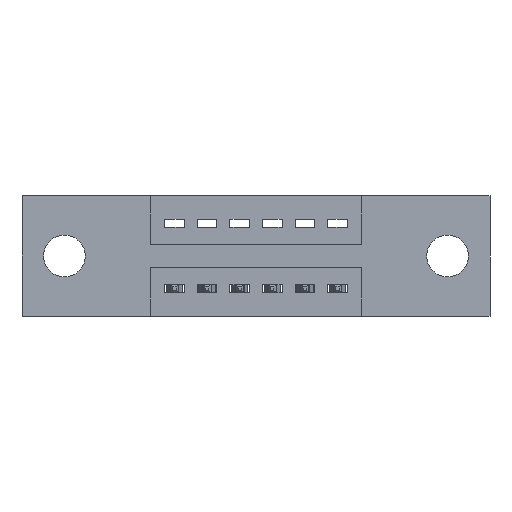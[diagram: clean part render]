
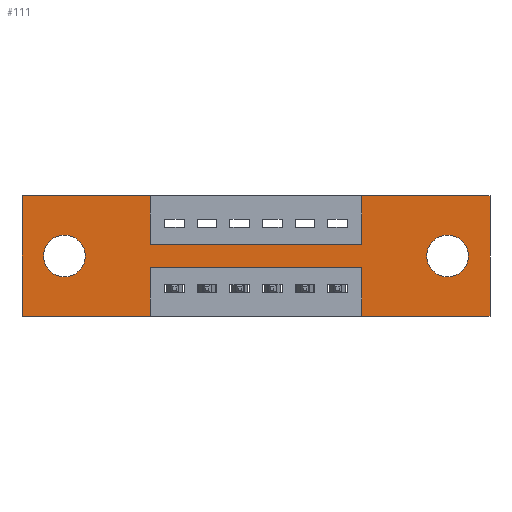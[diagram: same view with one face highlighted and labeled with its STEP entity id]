
A CAD part, front view. The second image highlights one B-rep face of the part: STEP entity #111.
In plain terms, the highlighted planar face has unit normal (0, -1, 0).
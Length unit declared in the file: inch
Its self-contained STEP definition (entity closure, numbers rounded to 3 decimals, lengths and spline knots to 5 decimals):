
#57 = VECTOR ( 'NONE', #6602, 39.37008 ) ;
#111 = ADVANCED_FACE ( 'NONE', ( #2194, #2697, #4175 ), #4312, .T. ) ;
#210 = VERTEX_POINT ( 'NONE', #6407 ) ;
#250 = ORIENTED_EDGE ( 'NONE', *, *, #3175, .F. ) ;
#259 = CARTESIAN_POINT ( 'NONE',  ( 0.13, 0., -0.249 ) ) ;
#515 = ORIENTED_EDGE ( 'NONE', *, *, #7250, .T. ) ;
#555 = DIRECTION ( 'NONE',  ( 0., 0., 1. ) ) ;
#652 = DIRECTION ( 'NONE',  ( 0., 0., -1. ) ) ;
#661 = DIRECTION ( 'NONE',  ( 0., 1., 0. ) ) ;
#688 = VERTEX_POINT ( 'NONE', #9074 ) ;
#694 = CARTESIAN_POINT ( 'NONE',  ( 1.305, 0., -0.185 ) ) ;
#770 = VERTEX_POINT ( 'NONE', #2885 ) ;
#778 = DIRECTION ( 'NONE',  ( 1., 0., 0. ) ) ;
#841 = CARTESIAN_POINT ( 'NONE',  ( 0., 0., 0. ) ) ;
#956 = VERTEX_POINT ( 'NONE', #259 ) ;
#989 = VECTOR ( 'NONE', #8501, 39.37008 ) ;
#998 = LINE ( 'NONE', #1547, #4602 ) ;
#1008 = VERTEX_POINT ( 'NONE', #4965 ) ;
#1047 = DIRECTION ( 'NONE',  ( -1., 0., 0. ) ) ;
#1071 = DIRECTION ( 'NONE',  ( 0., 0., -1. ) ) ;
#1086 = CARTESIAN_POINT ( 'NONE',  ( 1.435, 0., 0. ) ) ;
#1248 = CARTESIAN_POINT ( 'NONE',  ( 0., 0., -0.37 ) ) ;
#1488 = EDGE_LOOP ( 'NONE', ( #6995, #3356, #6456, #3856, #9124, #2241, #2354, #3052, #1968, #5906, #6136, #250 ) ) ;
#1507 = DIRECTION ( 'NONE',  ( 0., 1., 0. ) ) ;
#1532 = DIRECTION ( 'NONE',  ( -1., 0., 0. ) ) ;
#1547 = CARTESIAN_POINT ( 'NONE',  ( 0.3925, 0., -0.22 ) ) ;
#1750 = CARTESIAN_POINT ( 'NONE',  ( 1.0425, 0., -0.37 ) ) ;
#1777 = CARTESIAN_POINT ( 'NONE',  ( 0.3925, 0., -0.15 ) ) ;
#1778 = LINE ( 'NONE', #4325, #7411 ) ;
#1821 = DIRECTION ( 'NONE',  ( 1., 0., 0. ) ) ;
#1823 = CARTESIAN_POINT ( 'NONE',  ( 0., 0., 0. ) ) ;
#1830 = EDGE_CURVE ( 'NONE', #9375, #6815, #3980, .T. ) ;
#1839 = DIRECTION ( 'NONE',  ( 0., -1., 0. ) ) ;
#1924 = DIRECTION ( 'NONE',  ( 0., 1., 0. ) ) ;
#1968 = ORIENTED_EDGE ( 'NONE', *, *, #1830, .F. ) ;
#1976 = DIRECTION ( 'NONE',  ( 0., 0., 1. ) ) ;
#1982 = VECTOR ( 'NONE', #2106, 39.37008 ) ;
#2098 = CARTESIAN_POINT ( 'NONE',  ( 0.13, 0., -0.185 ) ) ;
#2106 = DIRECTION ( 'NONE',  ( 0., 0., -1. ) ) ;
#2166 = CARTESIAN_POINT ( 'NONE',  ( 0.3925, 0., 0. ) ) ;
#2194 = FACE_BOUND ( 'NONE', #7007, .T. ) ;
#2241 = ORIENTED_EDGE ( 'NONE', *, *, #5761, .F. ) ;
#2349 = CARTESIAN_POINT ( 'NONE',  ( 1.0425, 0., 0. ) ) ;
#2354 = ORIENTED_EDGE ( 'NONE', *, *, #4843, .F. ) ;
#2384 = EDGE_CURVE ( 'NONE', #6815, #3160, #4997, .T. ) ;
#2516 = CARTESIAN_POINT ( 'NONE',  ( 1.435, 0., -0.37 ) ) ;
#2584 = VECTOR ( 'NONE', #5367, 39.37008 ) ;
#2697 = FACE_BOUND ( 'NONE', #6129, .T. ) ;
#2764 = VERTEX_POINT ( 'NONE', #2937 ) ;
#2790 = CIRCLE ( 'NONE', #6164, 0.064 ) ;
#2824 = VECTOR ( 'NONE', #6377, 39.37008 ) ;
#2885 = CARTESIAN_POINT ( 'NONE',  ( 1.305, 0., -0.249 ) ) ;
#2937 = CARTESIAN_POINT ( 'NONE',  ( 0., 0., -0.37 ) ) ;
#3007 = EDGE_CURVE ( 'NONE', #7579, #4313, #6117, .T. ) ;
#3052 = ORIENTED_EDGE ( 'NONE', *, *, #2384, .F. ) ;
#3073 = EDGE_CURVE ( 'NONE', #770, #688, #3715, .T. ) ;
#3087 = LINE ( 'NONE', #7874, #989 ) ;
#3095 = VECTOR ( 'NONE', #1821, 39.37008 ) ;
#3103 = VECTOR ( 'NONE', #555, 39.37008 ) ;
#3120 = DIRECTION ( 'NONE',  ( 0., 0., -1. ) ) ;
#3160 = VERTEX_POINT ( 'NONE', #4500 ) ;
#3162 = VERTEX_POINT ( 'NONE', #4529 ) ;
#3175 = EDGE_CURVE ( 'NONE', #6709, #2764, #8242, .T. ) ;
#3309 = LINE ( 'NONE', #1823, #3095 ) ;
#3321 = VERTEX_POINT ( 'NONE', #5924 ) ;
#3356 = ORIENTED_EDGE ( 'NONE', *, *, #5820, .F. ) ;
#3430 = VERTEX_POINT ( 'NONE', #2349 ) ;
#3685 = DIRECTION ( 'NONE',  ( 0., 1., 0. ) ) ;
#3715 = CIRCLE ( 'NONE', #6693, 0.064 ) ;
#3856 = ORIENTED_EDGE ( 'NONE', *, *, #3007, .F. ) ;
#3952 = ORIENTED_EDGE ( 'NONE', *, *, #3073, .T. ) ;
#3980 = LINE ( 'NONE', #2166, #1982 ) ;
#3997 = VERTEX_POINT ( 'NONE', #4804 ) ;
#4112 = CARTESIAN_POINT ( 'NONE',  ( 0.3925, 0., 0. ) ) ;
#4127 = CARTESIAN_POINT ( 'NONE',  ( 1.0425, 0., -0.37 ) ) ;
#4175 = FACE_OUTER_BOUND ( 'NONE', #1488, .T. ) ;
#4291 = EDGE_CURVE ( 'NONE', #956, #3997, #2790, .T. ) ;
#4312 = PLANE ( 'NONE',  #7106 ) ;
#4313 = VERTEX_POINT ( 'NONE', #1750 ) ;
#4325 = CARTESIAN_POINT ( 'NONE',  ( 0., 0., 0. ) ) ;
#4349 = CARTESIAN_POINT ( 'NONE',  ( 0., 0., -0.37 ) ) ;
#4500 = CARTESIAN_POINT ( 'NONE',  ( 1.0425, 0., -0.15 ) ) ;
#4529 = CARTESIAN_POINT ( 'NONE',  ( 0.3925, 0., -0.22 ) ) ;
#4558 = CARTESIAN_POINT ( 'NONE',  ( 0., 0., -0.37 ) ) ;
#4602 = VECTOR ( 'NONE', #1532, 39.37008 ) ;
#4605 = AXIS2_PLACEMENT_3D ( 'NONE', #7954, #3685, #8582 ) ;
#4747 = DIRECTION ( 'NONE',  ( 0., 0., 1. ) ) ;
#4804 = CARTESIAN_POINT ( 'NONE',  ( 0.13, 0., -0.121 ) ) ;
#4843 = EDGE_CURVE ( 'NONE', #3160, #3430, #9267, .T. ) ;
#4965 = CARTESIAN_POINT ( 'NONE',  ( 0., 0., 0. ) ) ;
#4997 = LINE ( 'NONE', #6329, #2824 ) ;
#5065 = LINE ( 'NONE', #4127, #3103 ) ;
#5164 = VECTOR ( 'NONE', #778, 39.37008 ) ;
#5287 = EDGE_CURVE ( 'NONE', #2764, #1008, #1778, .T. ) ;
#5336 = EDGE_CURVE ( 'NONE', #4313, #3321, #5065, .T. ) ;
#5367 = DIRECTION ( 'NONE',  ( -1., 0., 0. ) ) ;
#5761 = EDGE_CURVE ( 'NONE', #3430, #210, #3309, .T. ) ;
#5820 = EDGE_CURVE ( 'NONE', #3321, #3162, #998, .T. ) ;
#5906 = ORIENTED_EDGE ( 'NONE', *, *, #6012, .F. ) ;
#5924 = CARTESIAN_POINT ( 'NONE',  ( 1.0425, 0., -0.22 ) ) ;
#5942 = EDGE_CURVE ( 'NONE', #210, #7579, #9336, .T. ) ;
#5984 = CARTESIAN_POINT ( 'NONE',  ( 1.305, 0., -0.185 ) ) ;
#6012 = EDGE_CURVE ( 'NONE', #1008, #9375, #7288, .T. ) ;
#6117 = LINE ( 'NONE', #1248, #9374 ) ;
#6129 = EDGE_LOOP ( 'NONE', ( #515, #6788 ) ) ;
#6136 = ORIENTED_EDGE ( 'NONE', *, *, #5287, .F. ) ;
#6164 = AXIS2_PLACEMENT_3D ( 'NONE', #2098, #1924, #1976 ) ;
#6295 = EDGE_CURVE ( 'NONE', #3162, #6709, #3087, .T. ) ;
#6329 = CARTESIAN_POINT ( 'NONE',  ( 0.3925, 0., -0.15 ) ) ;
#6349 = AXIS2_PLACEMENT_3D ( 'NONE', #5984, #1507, #6703 ) ;
#6377 = DIRECTION ( 'NONE',  ( 1., 0., 0. ) ) ;
#6407 = CARTESIAN_POINT ( 'NONE',  ( 1.435, 0., 0. ) ) ;
#6456 = ORIENTED_EDGE ( 'NONE', *, *, #5336, .F. ) ;
#6602 = DIRECTION ( 'NONE',  ( 0., 0., 1. ) ) ;
#6623 = CARTESIAN_POINT ( 'NONE',  ( 1.0425, 0., 0. ) ) ;
#6693 = AXIS2_PLACEMENT_3D ( 'NONE', #694, #661, #652 ) ;
#6703 = DIRECTION ( 'NONE',  ( 0., 0., -1. ) ) ;
#6709 = VERTEX_POINT ( 'NONE', #8168 ) ;
#6788 = ORIENTED_EDGE ( 'NONE', *, *, #4291, .T. ) ;
#6815 = VERTEX_POINT ( 'NONE', #1777 ) ;
#6995 = ORIENTED_EDGE ( 'NONE', *, *, #6295, .F. ) ;
#7007 = EDGE_LOOP ( 'NONE', ( #8629, #3952 ) ) ;
#7043 = CIRCLE ( 'NONE', #6349, 0.064 ) ;
#7106 = AXIS2_PLACEMENT_3D ( 'NONE', #4349, #1839, #3120 ) ;
#7250 = EDGE_CURVE ( 'NONE', #3997, #956, #8008, .T. ) ;
#7288 = LINE ( 'NONE', #841, #5164 ) ;
#7411 = VECTOR ( 'NONE', #4747, 39.37008 ) ;
#7505 = VECTOR ( 'NONE', #1071, 39.37008 ) ;
#7579 = VERTEX_POINT ( 'NONE', #2516 ) ;
#7874 = CARTESIAN_POINT ( 'NONE',  ( 0.3925, 0., -0.37 ) ) ;
#7954 = CARTESIAN_POINT ( 'NONE',  ( 0.13, 0., -0.185 ) ) ;
#8008 = CIRCLE ( 'NONE', #4605, 0.064 ) ;
#8134 = EDGE_CURVE ( 'NONE', #688, #770, #7043, .T. ) ;
#8168 = CARTESIAN_POINT ( 'NONE',  ( 0.3925, 0., -0.37 ) ) ;
#8242 = LINE ( 'NONE', #4558, #2584 ) ;
#8501 = DIRECTION ( 'NONE',  ( 0., 0., -1. ) ) ;
#8582 = DIRECTION ( 'NONE',  ( 0., 0., 1. ) ) ;
#8629 = ORIENTED_EDGE ( 'NONE', *, *, #8134, .T. ) ;
#9074 = CARTESIAN_POINT ( 'NONE',  ( 1.305, 0., -0.121 ) ) ;
#9124 = ORIENTED_EDGE ( 'NONE', *, *, #5942, .F. ) ;
#9267 = LINE ( 'NONE', #6623, #57 ) ;
#9336 = LINE ( 'NONE', #1086, #7505 ) ;
#9374 = VECTOR ( 'NONE', #1047, 39.37008 ) ;
#9375 = VERTEX_POINT ( 'NONE', #4112 ) ;
